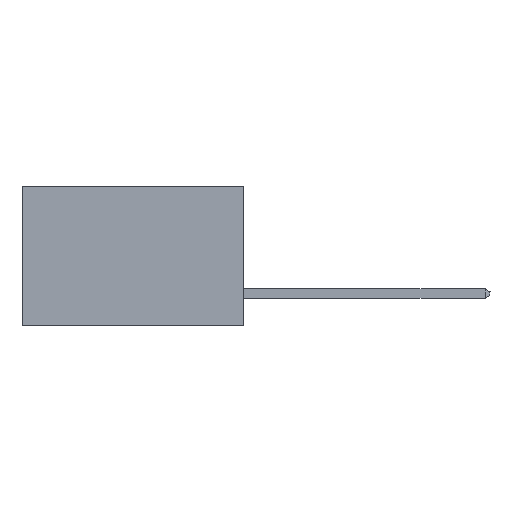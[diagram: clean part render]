
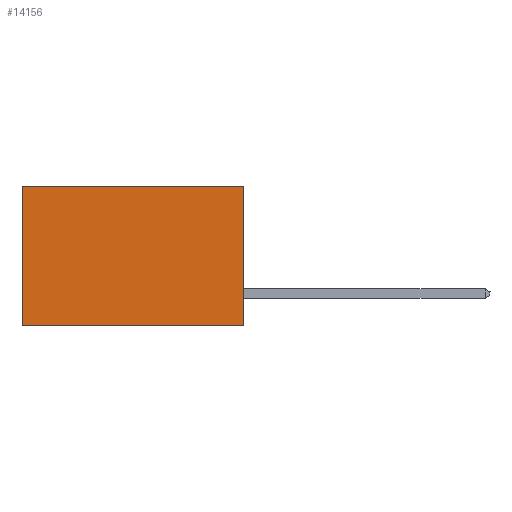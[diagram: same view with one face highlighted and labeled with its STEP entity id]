
A CAD part, left-side view. The second image highlights one B-rep face of the part: STEP entity #14156.
In plain terms, the highlighted planar face has unit normal (-1, 0, 0).
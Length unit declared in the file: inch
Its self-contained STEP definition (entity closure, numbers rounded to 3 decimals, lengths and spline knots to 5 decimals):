
#1215 = DIRECTION ( 'NONE',  ( 0., 1., 0. ) ) ;
#1462 = LINE ( 'NONE', #4947, #13519 ) ;
#1742 = CARTESIAN_POINT ( 'NONE',  ( 0.277, 0., 0. ) ) ;
#2114 = CARTESIAN_POINT ( 'NONE',  ( 0.277, 0.59, -0.37 ) ) ;
#2930 = DIRECTION ( 'NONE',  ( 0., 1., 0. ) ) ;
#2945 = DIRECTION ( 'NONE',  ( 0., 0., -1. ) ) ;
#3121 = VECTOR ( 'NONE', #2930, 39.37008 ) ;
#3214 = CARTESIAN_POINT ( 'NONE',  ( 0.277, 0., -0.37 ) ) ;
#3445 = EDGE_CURVE ( 'NONE', #15135, #8929, #1462, .T. ) ;
#4307 = ORIENTED_EDGE ( 'NONE', *, *, #3445, .T. ) ;
#4947 = CARTESIAN_POINT ( 'NONE',  ( 0.277, 0.59, -0.37 ) ) ;
#5034 = LINE ( 'NONE', #7218, #10944 ) ;
#5133 = EDGE_CURVE ( 'NONE', #14482, #15135, #7055, .T. ) ;
#5796 = CARTESIAN_POINT ( 'NONE',  ( 0.277, 0., 0. ) ) ;
#7055 = LINE ( 'NONE', #1742, #3121 ) ;
#7218 = CARTESIAN_POINT ( 'NONE',  ( 0.277, 0., -0.37 ) ) ;
#7912 = ORIENTED_EDGE ( 'NONE', *, *, #11050, .F. ) ;
#8929 = VERTEX_POINT ( 'NONE', #2114 ) ;
#8961 = EDGE_CURVE ( 'NONE', #12808, #8929, #5034, .T. ) ;
#9526 = AXIS2_PLACEMENT_3D ( 'NONE', #11161, #10040, #2945 ) ;
#10040 = DIRECTION ( 'NONE',  ( 1., 0., 0. ) ) ;
#10944 = VECTOR ( 'NONE', #1215, 39.37008 ) ;
#10960 = ORIENTED_EDGE ( 'NONE', *, *, #5133, .T. ) ;
#11050 = EDGE_CURVE ( 'NONE', #14482, #12808, #12477, .T. ) ;
#11161 = CARTESIAN_POINT ( 'NONE',  ( 0.277, 0., -0.37 ) ) ;
#11994 = CARTESIAN_POINT ( 'NONE',  ( 0.277, 0., -0.37 ) ) ;
#12138 = VECTOR ( 'NONE', #13094, 39.37008 ) ;
#12477 = LINE ( 'NONE', #11994, #12138 ) ;
#12576 = FACE_OUTER_BOUND ( 'NONE', #14182, .T. ) ;
#12808 = VERTEX_POINT ( 'NONE', #3214 ) ;
#12836 = CARTESIAN_POINT ( 'NONE',  ( 0.277, 0.59, 0. ) ) ;
#13094 = DIRECTION ( 'NONE',  ( 0., 0., -1. ) ) ;
#13519 = VECTOR ( 'NONE', #14829, 39.37008 ) ;
#13552 = ORIENTED_EDGE ( 'NONE', *, *, #8961, .F. ) ;
#14156 = ADVANCED_FACE ( 'NONE', ( #12576 ), #14439, .F. ) ;
#14182 = EDGE_LOOP ( 'NONE', ( #4307, #13552, #7912, #10960 ) ) ;
#14439 = PLANE ( 'NONE',  #9526 ) ;
#14482 = VERTEX_POINT ( 'NONE', #5796 ) ;
#14829 = DIRECTION ( 'NONE',  ( 0., 0., -1. ) ) ;
#15135 = VERTEX_POINT ( 'NONE', #12836 ) ;
